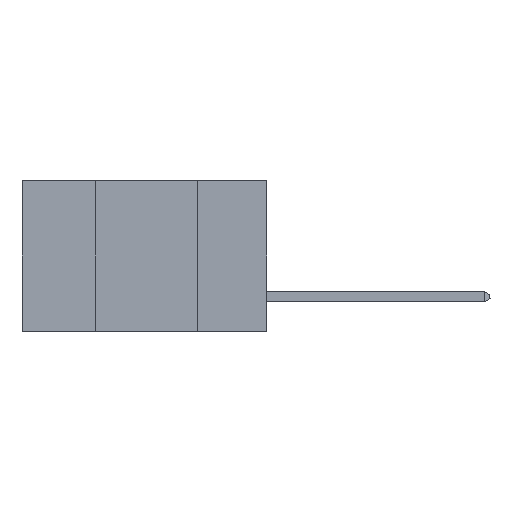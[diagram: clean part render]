
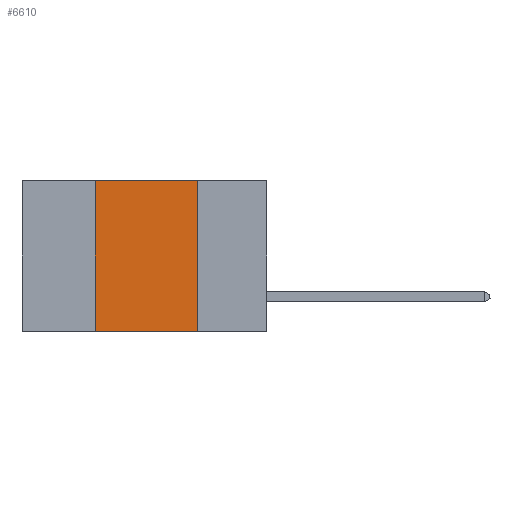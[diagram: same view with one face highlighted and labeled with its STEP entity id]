
A CAD part, left-side view. The second image highlights one B-rep face of the part: STEP entity #6610.
In plain terms, the highlighted planar face has unit normal (-1, 0, 0).
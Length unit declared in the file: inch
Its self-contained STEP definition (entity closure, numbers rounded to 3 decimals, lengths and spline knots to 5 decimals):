
#158 = LINE ( 'NONE', #4640, #7520 ) ;
#738 = PLANE ( 'NONE',  #10643 ) ;
#1364 = CARTESIAN_POINT ( 'NONE',  ( 0., 0.42, -0.37 ) ) ;
#1918 = VERTEX_POINT ( 'NONE', #1364 ) ;
#1952 = CARTESIAN_POINT ( 'NONE',  ( 0., 0.17, 0. ) ) ;
#2213 = EDGE_CURVE ( 'NONE', #3636, #4969, #9923, .T. ) ;
#2555 = ORIENTED_EDGE ( 'NONE', *, *, #10968, .F. ) ;
#2800 = VECTOR ( 'NONE', #5601, 39.37008 ) ;
#2855 = CARTESIAN_POINT ( 'NONE',  ( 0., 0.17, -0.37 ) ) ;
#3613 = DIRECTION ( 'NONE',  ( 1., 0., 0. ) ) ;
#3636 = VERTEX_POINT ( 'NONE', #9616 ) ;
#3702 = FACE_OUTER_BOUND ( 'NONE', #5246, .T. ) ;
#3959 = CARTESIAN_POINT ( 'NONE',  ( 0., 0.42, 0. ) ) ;
#4513 = DIRECTION ( 'NONE',  ( 0., -1., 0. ) ) ;
#4581 = CARTESIAN_POINT ( 'NONE',  ( 0., 0.6, 0. ) ) ;
#4640 = CARTESIAN_POINT ( 'NONE',  ( 0., 0.6, 0. ) ) ;
#4969 = VERTEX_POINT ( 'NONE', #2855 ) ;
#5246 = EDGE_LOOP ( 'NONE', ( #9453, #7861, #2555, #7544 ) ) ;
#5601 = DIRECTION ( 'NONE',  ( 0., 0., -1. ) ) ;
#6610 = ADVANCED_FACE ( 'NONE', ( #3702 ), #738, .F. ) ;
#7162 = VECTOR ( 'NONE', #11537, 39.37008 ) ;
#7478 = VECTOR ( 'NONE', #9393, 39.37008 ) ;
#7520 = VECTOR ( 'NONE', #4513, 39.37008 ) ;
#7544 = ORIENTED_EDGE ( 'NONE', *, *, #11017, .T. ) ;
#7748 = CARTESIAN_POINT ( 'NONE',  ( 0., 0.42, 0. ) ) ;
#7861 = ORIENTED_EDGE ( 'NONE', *, *, #9769, .F. ) ;
#7943 = CARTESIAN_POINT ( 'NONE',  ( 0., 0.6, -0.37 ) ) ;
#9393 = DIRECTION ( 'NONE',  ( 0., 0., 1. ) ) ;
#9453 = ORIENTED_EDGE ( 'NONE', *, *, #2213, .F. ) ;
#9616 = CARTESIAN_POINT ( 'NONE',  ( 0., 0.17, 0. ) ) ;
#9688 = LINE ( 'NONE', #7943, #7162 ) ;
#9769 = EDGE_CURVE ( 'NONE', #11650, #3636, #158, .T. ) ;
#9923 = LINE ( 'NONE', #1952, #2800 ) ;
#10643 = AXIS2_PLACEMENT_3D ( 'NONE', #4581, #3613, #11073 ) ;
#10968 = EDGE_CURVE ( 'NONE', #1918, #11650, #11121, .T. ) ;
#11017 = EDGE_CURVE ( 'NONE', #1918, #4969, #9688, .T. ) ;
#11073 = DIRECTION ( 'NONE',  ( 0., 0., -1. ) ) ;
#11121 = LINE ( 'NONE', #3959, #7478 ) ;
#11537 = DIRECTION ( 'NONE',  ( 0., -1., 0. ) ) ;
#11650 = VERTEX_POINT ( 'NONE', #7748 ) ;
